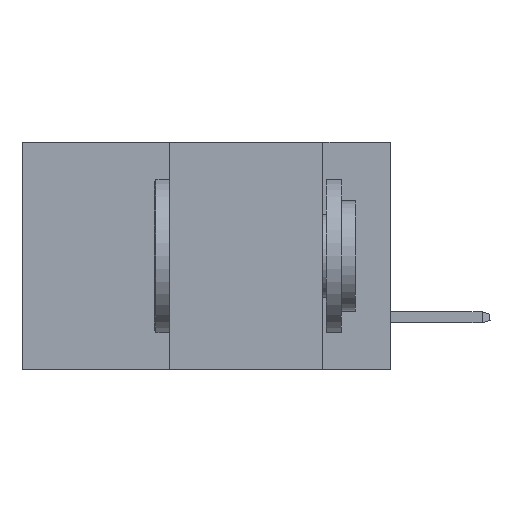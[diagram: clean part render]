
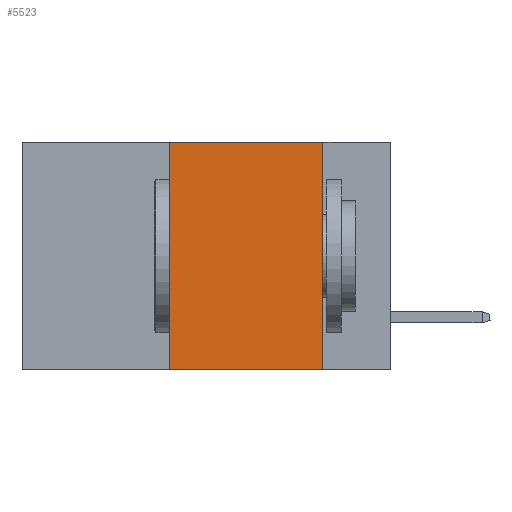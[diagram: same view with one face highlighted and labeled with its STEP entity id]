
A CAD part, left-side view. The second image highlights one B-rep face of the part: STEP entity #5523.
In plain terms, the highlighted planar face has unit normal (-1, 0, 0).
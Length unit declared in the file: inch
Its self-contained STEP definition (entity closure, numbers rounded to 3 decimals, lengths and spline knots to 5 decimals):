
#1392 = LINE ( 'NONE', #36521, #32946 ) ;
#2486 = DIRECTION ( 'NONE',  ( 0., 0., 1. ) ) ;
#4963 = ORIENTED_EDGE ( 'NONE', *, *, #19330, .F. ) ;
#5523 = ADVANCED_FACE ( 'NONE', ( #27266 ), #16441, .F. ) ;
#5670 = CARTESIAN_POINT ( 'NONE',  ( 0., 0.6, 0. ) ) ;
#5959 = DIRECTION ( 'NONE',  ( 0., -1., 0. ) ) ;
#5974 = LINE ( 'NONE', #35947, #16084 ) ;
#7272 = VERTEX_POINT ( 'NONE', #18331 ) ;
#7419 = CARTESIAN_POINT ( 'NONE',  ( 0., 0.6, 0. ) ) ;
#7487 = VECTOR ( 'NONE', #39408, 39.37008 ) ;
#8094 = VERTEX_POINT ( 'NONE', #38824 ) ;
#11360 = VERTEX_POINT ( 'NONE', #40768 ) ;
#12748 = EDGE_CURVE ( 'NONE', #11360, #8094, #5974, .T. ) ;
#13060 = LINE ( 'NONE', #7419, #13535 ) ;
#13535 = VECTOR ( 'NONE', #5959, 39.37008 ) ;
#15821 = DIRECTION ( 'NONE',  ( 0., -1., 0. ) ) ;
#16084 = VECTOR ( 'NONE', #15821, 39.37008 ) ;
#16441 = PLANE ( 'NONE',  #42566 ) ;
#16640 = LINE ( 'NONE', #39715, #7487 ) ;
#18190 = ORIENTED_EDGE ( 'NONE', *, *, #12748, .T. ) ;
#18331 = CARTESIAN_POINT ( 'NONE',  ( 0., 0.11, 0. ) ) ;
#19330 = EDGE_CURVE ( 'NONE', #11360, #32609, #1392, .T. ) ;
#23299 = DIRECTION ( 'NONE',  ( 1., 0., 0. ) ) ;
#27187 = CARTESIAN_POINT ( 'NONE',  ( 0., 0.36, 0. ) ) ;
#27266 = FACE_OUTER_BOUND ( 'NONE', #44165, .T. ) ;
#27821 = ORIENTED_EDGE ( 'NONE', *, *, #36162, .F. ) ;
#28133 = EDGE_CURVE ( 'NONE', #7272, #8094, #16640, .T. ) ;
#29579 = DIRECTION ( 'NONE',  ( 0., 0., -1. ) ) ;
#32609 = VERTEX_POINT ( 'NONE', #27187 ) ;
#32946 = VECTOR ( 'NONE', #2486, 39.37008 ) ;
#35938 = ORIENTED_EDGE ( 'NONE', *, *, #28133, .F. ) ;
#35947 = CARTESIAN_POINT ( 'NONE',  ( 0., 0.6, -0.37 ) ) ;
#36162 = EDGE_CURVE ( 'NONE', #32609, #7272, #13060, .T. ) ;
#36521 = CARTESIAN_POINT ( 'NONE',  ( 0., 0.36, 0. ) ) ;
#38824 = CARTESIAN_POINT ( 'NONE',  ( 0., 0.11, -0.37 ) ) ;
#39408 = DIRECTION ( 'NONE',  ( 0., 0., -1. ) ) ;
#39715 = CARTESIAN_POINT ( 'NONE',  ( 0., 0.11, 0. ) ) ;
#40768 = CARTESIAN_POINT ( 'NONE',  ( 0., 0.36, -0.37 ) ) ;
#42566 = AXIS2_PLACEMENT_3D ( 'NONE', #5670, #23299, #29579 ) ;
#44165 = EDGE_LOOP ( 'NONE', ( #35938, #27821, #4963, #18190 ) ) ;
